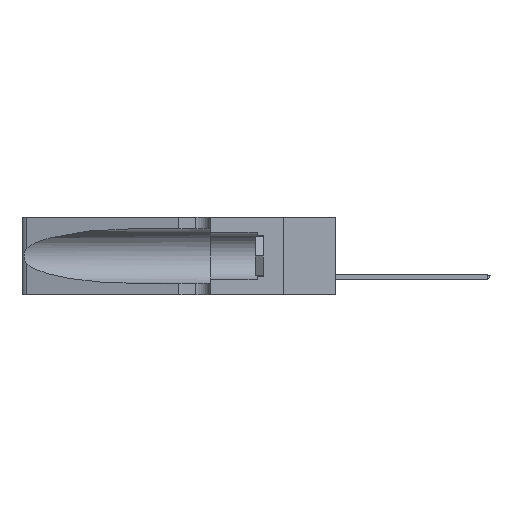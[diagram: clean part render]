
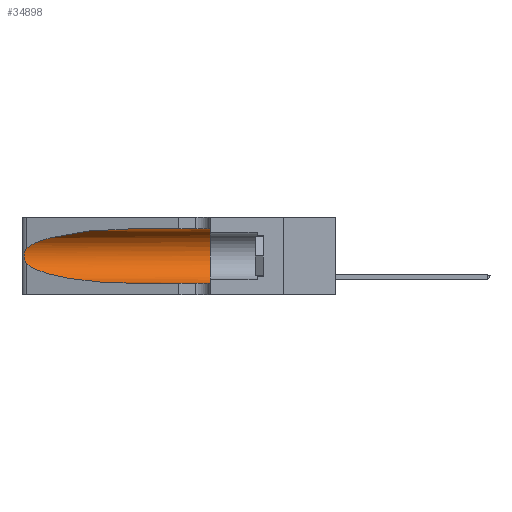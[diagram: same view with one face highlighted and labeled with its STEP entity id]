
A CAD part, left-side view. The second image highlights one B-rep face of the part: STEP entity #34898.
In plain terms, the highlighted cylindrical face has radius 3.308 mm (diameter 6.617 mm), a partial arc.
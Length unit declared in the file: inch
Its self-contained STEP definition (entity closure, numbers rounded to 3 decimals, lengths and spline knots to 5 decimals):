
#883 = VERTEX_POINT ( 'NONE', #19548 ) ;
#907 = VECTOR ( 'NONE', #38197, 39.37008 ) ;
#1112 = EDGE_LOOP ( 'NONE', ( #18928, #20938, #35378, #32671, #40375, #10475 ) ) ;
#2197 = FACE_OUTER_BOUND ( 'NONE', #1112, .T. ) ;
#2559 = CARTESIAN_POINT ( 'NONE',  ( 0.1305, 1.61858, 0.05475 ) ) ;
#3160 = CARTESIAN_POINT ( 'NONE',  ( 0.26075, 1.23896, 0.19203 ) ) ;
#4850 = CARTESIAN_POINT ( 'NONE',  ( 0.1305, 0.35, 0.185 ) ) ;
#4865 = VECTOR ( 'NONE', #20428, 39.37008 ) ;
#5368 = EDGE_CURVE ( 'NONE', #30169, #35243, #9592, .T. ) ;
#6097 = VERTEX_POINT ( 'NONE', #34357 ) ;
#6810 = CARTESIAN_POINT ( 'NONE',  ( 0.25555, 1.22993, 0.14849 ) ) ;
#9029 = CARTESIAN_POINT ( 'NONE',  ( 0.2373, 1.15595, 0.08982 ) ) ;
#9289 = CIRCLE ( 'NONE', #40362, 0.13025 ) ;
#9592 =( BOUNDED_CURVE ( )  B_SPLINE_CURVE ( 3, ( #32145, #22600, #35465, #13162 ),
 .UNSPECIFIED., .F., .F. ) 
 B_SPLINE_CURVE_WITH_KNOTS ( ( 4, 4 ),
 ( 1.5708, 2.84003 ),
 .UNSPECIFIED. ) 
 CURVE ( )  GEOMETRIC_REPRESENTATION_ITEM ( )  RATIONAL_B_SPLINE_CURVE ( ( 1., 0.87, 0.87, 1. ) ) 
 REPRESENTATION_ITEM ( '' )  );
#10475 = ORIENTED_EDGE ( 'NONE', *, *, #33292, .F. ) ;
#10570 = DIRECTION ( 'NONE',  ( 0., -1., 0. ) ) ;
#11379 = VERTEX_POINT ( 'NONE', #17184 ) ;
#11466 = DIRECTION ( 'NONE',  ( 0., 1., 0. ) ) ;
#13162 = CARTESIAN_POINT ( 'NONE',  ( 0.25487, 1.22718, 0.22369 ) ) ;
#14135 =( BOUNDED_CURVE ( )  B_SPLINE_CURVE ( 3, ( #18688, #9029, #37923, #22044 ),
 .UNSPECIFIED., .F., .T. ) 
 B_SPLINE_CURVE_WITH_KNOTS ( ( 4, 4 ),
 ( 3.44316, 4.71239 ),
 .UNSPECIFIED. ) 
 CURVE ( )  GEOMETRIC_REPRESENTATION_ITEM ( )  RATIONAL_B_SPLINE_CURVE ( ( 1., 0.87, 0.87, 1. ) ) 
 REPRESENTATION_ITEM ( '' )  );
#14878 = EDGE_CURVE ( 'NONE', #6097, #883, #9289, .T. ) ;
#14962 = CARTESIAN_POINT ( 'NONE',  ( 0.25639, 1.23184, 0.21858 ) ) ;
#15059 = LINE ( 'NONE', #2559, #907 ) ;
#16085 = CARTESIAN_POINT ( 'NONE',  ( 0.25787, 1.23484, 0.2124 ) ) ;
#17184 = CARTESIAN_POINT ( 'NONE',  ( 0.25487, 1.22718, 0.14631 ) ) ;
#18015 = EDGE_CURVE ( 'NONE', #35243, #11379, #40699, .T. ) ;
#18688 = CARTESIAN_POINT ( 'NONE',  ( 0.25487, 1.22718, 0.14631 ) ) ;
#18928 = ORIENTED_EDGE ( 'NONE', *, *, #5368, .T. ) ;
#19521 = CARTESIAN_POINT ( 'NONE',  ( 0.25487, 1.22718, 0.22369 ) ) ;
#19548 = CARTESIAN_POINT ( 'NONE',  ( 0.1305, 0.35, 0.05475 ) ) ;
#20428 = DIRECTION ( 'NONE',  ( 0., -1., 0. ) ) ;
#20938 = ORIENTED_EDGE ( 'NONE', *, *, #18015, .T. ) ;
#22044 = CARTESIAN_POINT ( 'NONE',  ( 0.1305, 0.72297, 0.05475 ) ) ;
#22401 = CARTESIAN_POINT ( 'NONE',  ( 0.26018, 1.23835, 0.19895 ) ) ;
#22600 = CARTESIAN_POINT ( 'NONE',  ( 0.18966, 0.96281, 0.31525 ) ) ;
#23166 = CARTESIAN_POINT ( 'NONE',  ( 0.25487, 1.22718, 0.14631 ) ) ;
#24509 = DIRECTION ( 'NONE',  ( 0., 0., 1. ) ) ;
#25116 = CARTESIAN_POINT ( 'NONE',  ( 0.1305, 0.72297, 0.05475 ) ) ;
#25260 = CARTESIAN_POINT ( 'NONE',  ( 0.25856, 1.23593, 0.16098 ) ) ;
#25411 = CARTESIAN_POINT ( 'NONE',  ( 0.25854, 1.2359, 0.20912 ) ) ;
#25422 = AXIS2_PLACEMENT_3D ( 'NONE', #30075, #10570, #33297 ) ;
#27916 = CARTESIAN_POINT ( 'NONE',  ( 0.25555, 1.22994, 0.2215 ) ) ;
#30075 = CARTESIAN_POINT ( 'NONE',  ( 0.1305, 1.61858, 0.185 ) ) ;
#30169 = VERTEX_POINT ( 'NONE', #34733 ) ;
#31511 = EDGE_CURVE ( 'NONE', #36513, #883, #15059, .T. ) ;
#32145 = CARTESIAN_POINT ( 'NONE',  ( 0.1305, 0.72297, 0.31525 ) ) ;
#32202 = CARTESIAN_POINT ( 'NONE',  ( 0.26017, 1.23833, 0.17102 ) ) ;
#32600 = EDGE_CURVE ( 'NONE', #11379, #36513, #14135, .T. ) ;
#32671 = ORIENTED_EDGE ( 'NONE', *, *, #31511, .T. ) ;
#33292 = EDGE_CURVE ( 'NONE', #30169, #6097, #38483, .T. ) ;
#33297 = DIRECTION ( 'NONE',  ( 0., 0., -1. ) ) ;
#33819 = CYLINDRICAL_SURFACE ( 'NONE', #25422, 0.13025 ) ;
#34357 = CARTESIAN_POINT ( 'NONE',  ( 0.1305, 0.35, 0.31525 ) ) ;
#34733 = CARTESIAN_POINT ( 'NONE',  ( 0.1305, 0.72297, 0.31525 ) ) ;
#34898 = ADVANCED_FACE ( 'NONE', ( #2197 ), #33819, .F. ) ;
#35243 = VERTEX_POINT ( 'NONE', #19521 ) ;
#35378 = ORIENTED_EDGE ( 'NONE', *, *, #32600, .T. ) ;
#35465 = CARTESIAN_POINT ( 'NONE',  ( 0.2373, 1.15595, 0.28018 ) ) ;
#35915 = CARTESIAN_POINT ( 'NONE',  ( 0.25639, 1.23186, 0.15144 ) ) ;
#36417 = CARTESIAN_POINT ( 'NONE',  ( 0.1305, 1.61858, 0.31525 ) ) ;
#36513 = VERTEX_POINT ( 'NONE', #25116 ) ;
#37854 = CARTESIAN_POINT ( 'NONE',  ( 0.25487, 1.22718, 0.22369 ) ) ;
#37923 = CARTESIAN_POINT ( 'NONE',  ( 0.18966, 0.96281, 0.05475 ) ) ;
#38197 = DIRECTION ( 'NONE',  ( 0., -1., 0. ) ) ;
#38251 = CARTESIAN_POINT ( 'NONE',  ( 0.26075, 1.23896, 0.178 ) ) ;
#38483 = LINE ( 'NONE', #36417, #4865 ) ;
#40362 = AXIS2_PLACEMENT_3D ( 'NONE', #4850, #11466, #24509 ) ;
#40375 = ORIENTED_EDGE ( 'NONE', *, *, #14878, .F. ) ;
#40699 = B_SPLINE_CURVE_WITH_KNOTS ( 'NONE', 3,
 ( #37854, #27916, #14962, #16085, #25411, #22401, #3160, #38251, #32202, #25260, #41478, #35915, #6810, #23166 ),
 .UNSPECIFIED., .F., .F.,
 ( 4, 2, 2, 2, 2, 2, 4 ),
 ( 0., 0.00027, 0.00053, 0.00107, 0.0016, 0.00187, 0.00214 ),
 .UNSPECIFIED. ) ;
#41478 = CARTESIAN_POINT ( 'NONE',  ( 0.25789, 1.23486, 0.15765 ) ) ;
